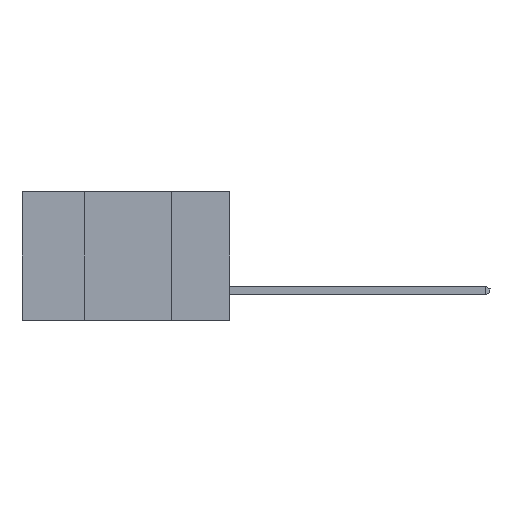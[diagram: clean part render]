
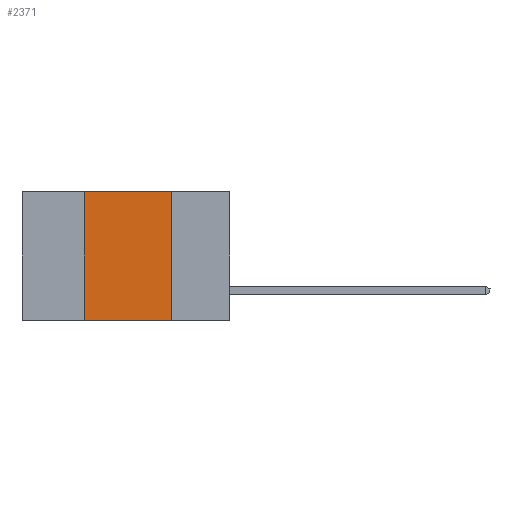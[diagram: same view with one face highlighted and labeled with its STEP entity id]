
A CAD part, left-side view. The second image highlights one B-rep face of the part: STEP entity #2371.
In plain terms, the highlighted planar face has unit normal (-1, 0, 0).
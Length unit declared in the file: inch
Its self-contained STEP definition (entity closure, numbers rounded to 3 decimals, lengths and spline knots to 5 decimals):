
#1 = LINE ( 'NONE', #11992, #12821 ) ;
#406 = DIRECTION ( 'NONE',  ( 0., 0., 1. ) ) ;
#2117 = EDGE_CURVE ( 'NONE', #11653, #10051, #1, .T. ) ;
#2278 = EDGE_CURVE ( 'NONE', #9671, #12028, #9863, .T. ) ;
#2371 = ADVANCED_FACE ( 'NONE', ( #3461 ), #15255, .F. ) ;
#2799 = CARTESIAN_POINT ( 'NONE',  ( 0., 0.42, -0.37 ) ) ;
#3014 = ORIENTED_EDGE ( 'NONE', *, *, #2117, .F. ) ;
#3461 = FACE_OUTER_BOUND ( 'NONE', #4377, .T. ) ;
#4046 = DIRECTION ( 'NONE',  ( 0., -1., 0. ) ) ;
#4361 = DIRECTION ( 'NONE',  ( 1., 0., 0. ) ) ;
#4377 = EDGE_LOOP ( 'NONE', ( #11107, #3014, #12934, #5104 ) ) ;
#4921 = DIRECTION ( 'NONE',  ( 0., -1., 0. ) ) ;
#5104 = ORIENTED_EDGE ( 'NONE', *, *, #2278, .T. ) ;
#5410 = CARTESIAN_POINT ( 'NONE',  ( 0., 0.17, -0.37 ) ) ;
#5588 = CARTESIAN_POINT ( 'NONE',  ( 0., 0.42, 0. ) ) ;
#5729 = AXIS2_PLACEMENT_3D ( 'NONE', #8308, #4361, #11744 ) ;
#6025 = CARTESIAN_POINT ( 'NONE',  ( 0., 0.42, -0.37 ) ) ;
#6627 = CARTESIAN_POINT ( 'NONE',  ( 0., 0.17, -0.37 ) ) ;
#8308 = CARTESIAN_POINT ( 'NONE',  ( 0., 0.6, 0. ) ) ;
#9277 = CARTESIAN_POINT ( 'NONE',  ( 0., 0.17, 0. ) ) ;
#9579 = VECTOR ( 'NONE', #12574, 39.37008 ) ;
#9671 = VERTEX_POINT ( 'NONE', #6025 ) ;
#9863 = LINE ( 'NONE', #11038, #10783 ) ;
#10051 = VERTEX_POINT ( 'NONE', #9277 ) ;
#10124 = LINE ( 'NONE', #6627, #9579 ) ;
#10783 = VECTOR ( 'NONE', #4046, 39.37008 ) ;
#10862 = EDGE_CURVE ( 'NONE', #10051, #12028, #10124, .T. ) ;
#11038 = CARTESIAN_POINT ( 'NONE',  ( 0., 0.6, -0.37 ) ) ;
#11107 = ORIENTED_EDGE ( 'NONE', *, *, #10862, .F. ) ;
#11653 = VERTEX_POINT ( 'NONE', #5588 ) ;
#11744 = DIRECTION ( 'NONE',  ( 0., 0., -1. ) ) ;
#11992 = CARTESIAN_POINT ( 'NONE',  ( 0., 0.6, 0. ) ) ;
#12028 = VERTEX_POINT ( 'NONE', #5410 ) ;
#12287 = VECTOR ( 'NONE', #406, 39.37008 ) ;
#12574 = DIRECTION ( 'NONE',  ( 0., 0., -1. ) ) ;
#12821 = VECTOR ( 'NONE', #4921, 39.37008 ) ;
#12934 = ORIENTED_EDGE ( 'NONE', *, *, #15035, .F. ) ;
#13931 = LINE ( 'NONE', #2799, #12287 ) ;
#15035 = EDGE_CURVE ( 'NONE', #9671, #11653, #13931, .T. ) ;
#15255 = PLANE ( 'NONE',  #5729 ) ;
